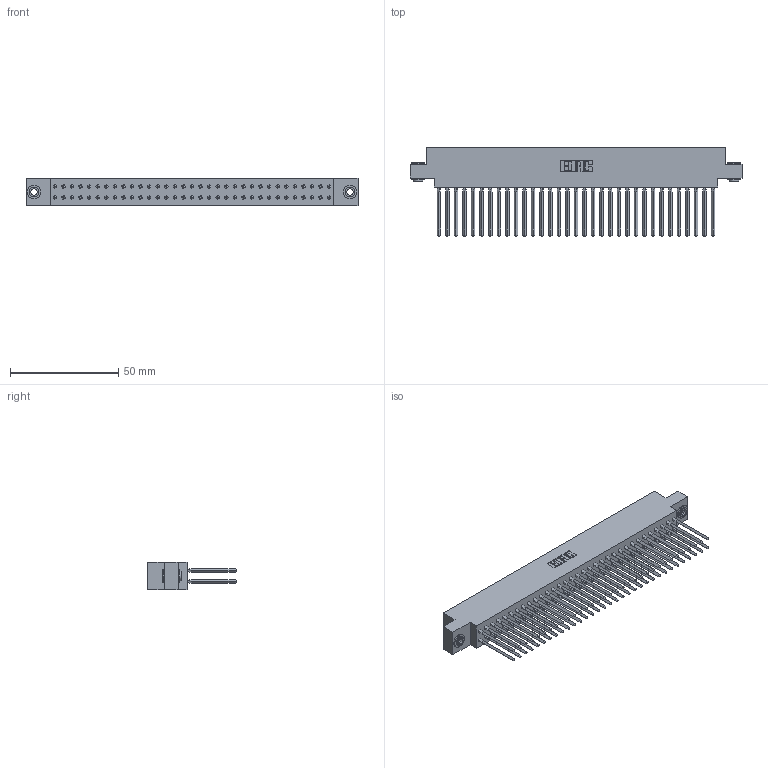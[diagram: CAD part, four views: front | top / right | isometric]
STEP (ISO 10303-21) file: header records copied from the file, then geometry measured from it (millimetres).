
FILE_DESCRIPTION (( 'STEP AP203' ), '1' );
FILE_NAME ('317-066-543-803.STEP', '2020-02-28T06:25:35', ( '' ), ( '' ), 'SwSTEP 2.0', 'SolidWorks 2016', '' );
FILE_SCHEMA (( 'CONFIG_CONTROL_DESIGN' ));
Length unit declared in the file: inch
Products named in the file (4): 317 Part_.156 Dia - TH; 317-066-543-803; 317-290-001_543; 345-250-002_345-250-002-102
Assembly tree (69 placements, depth 2):
  317-066-543-803
    317 Part_.156 Dia - TH
    317-290-001_543  x66
    345-250-002_345-250-002-102  x2
Bounding box: 153.47 x 41.15 x 12.7 mm (x, y, z)
Volume: 25800.1 mm3; surface area: 38998.9 mm2
Topology: 69 solids, 69 shells, 6014 faces, 16653 edges, 10724 vertices
Faces by surface type: plane 4886, cylinder 856, bspline 264, cone 8
Entity records: 49607 total; most frequent: CARTESIAN_POINT 9038, ORIENTED_EDGE 8530, DIRECTION 7157, EDGE_CURVE 4265, VECTOR 3985, LINE 3985, VERTEX_POINT 2835, AXIS2_PLACEMENT_3D 1586
